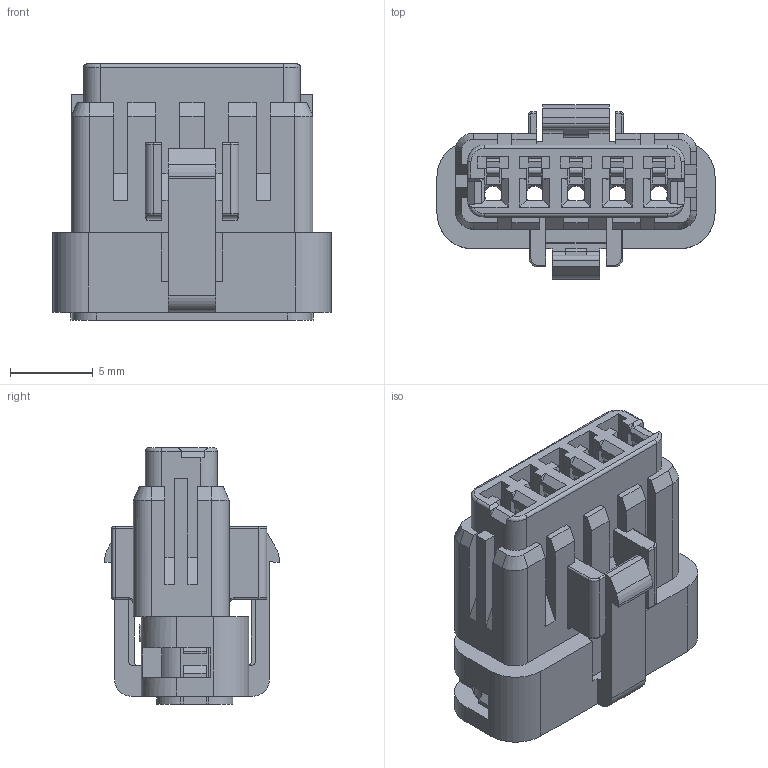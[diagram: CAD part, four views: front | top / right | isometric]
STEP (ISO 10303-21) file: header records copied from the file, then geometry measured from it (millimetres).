
FILE_DESCRIPTION (( 'STEP AP203' ), '1' );
FILE_NAME ('560-005-000-611.STEP', '2020-07-24T15:38:58', ( '' ), ( '' ), 'SwSTEP 2.0', 'SolidWorks 2020', '' );
FILE_SCHEMA (( 'CONFIG_CONTROL_DESIGN' ));
Length unit declared in the file: millimetre
Products named in the file (5): FEMALE_HOUSING_5POS_ORANGE; 560-005-000-611; REAR-GASKET-5POS_ORANGE; REAR-INSULATOR-5POS-1
Assembly tree (4 placements, depth 3):
  560-005-000-611
    560-005-000-611
      FEMALE_HOUSING_5POS_ORANGE
      REAR-GASKET-5POS_ORANGE
      REAR-INSULATOR-5POS-1
Bounding box: 16.8 x 10.55 x 15.48 mm (x, y, z)
Volume: 1037.2 mm3; surface area: 2490.6 mm2
Topology: 3 solids, 3 shells, 936 faces, 2514 edges, 1586 vertices
Faces by surface type: plane 560, cylinder 172, torus 104, cone 100
Entity records: 29589 total; most frequent: CARTESIAN_POINT 5370, ORIENTED_EDGE 5028, DIRECTION 4904, EDGE_CURVE 2514, LINE 1820, VECTOR 1820, VERTEX_POINT 1586, AXIS2_PLACEMENT_3D 1542
